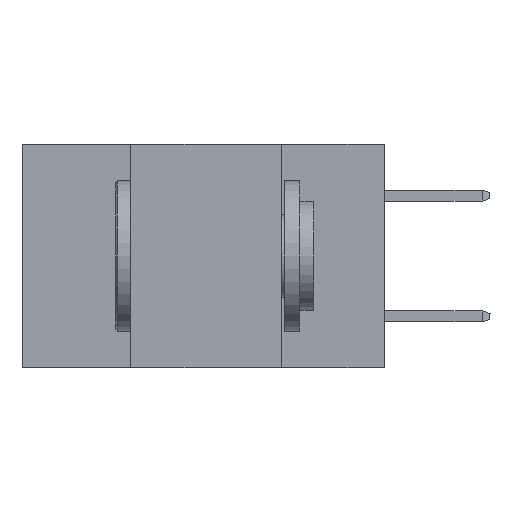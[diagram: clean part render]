
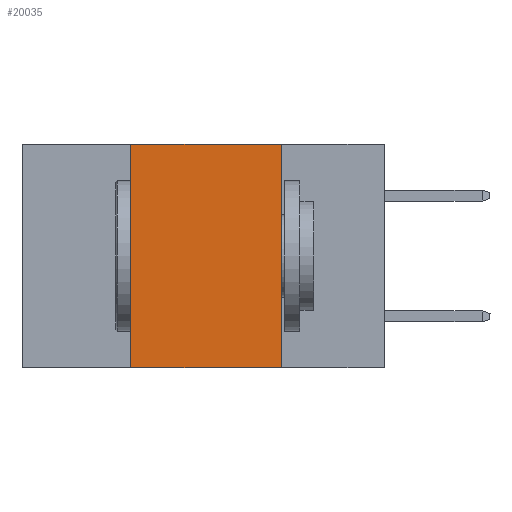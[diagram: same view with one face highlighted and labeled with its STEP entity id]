
A CAD part, left-side view. The second image highlights one B-rep face of the part: STEP entity #20035.
In plain terms, the highlighted planar face has unit normal (-1, 0, 0).
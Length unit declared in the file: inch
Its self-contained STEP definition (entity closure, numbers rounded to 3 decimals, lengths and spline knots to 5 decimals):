
#351 = VERTEX_POINT ( 'NONE', #7982 ) ;
#1203 = PLANE ( 'NONE',  #13184 ) ;
#2662 = DIRECTION ( 'NONE',  ( 0., 0., -1. ) ) ;
#3090 = CARTESIAN_POINT ( 'NONE',  ( 0., 0.6, 0. ) ) ;
#3167 = DIRECTION ( 'NONE',  ( 1., 0., 0. ) ) ;
#3627 = VERTEX_POINT ( 'NONE', #15160 ) ;
#3742 = CARTESIAN_POINT ( 'NONE',  ( 0., 0.6, 0. ) ) ;
#4454 = EDGE_CURVE ( 'NONE', #16259, #22683, #21124, .T. ) ;
#4916 = EDGE_LOOP ( 'NONE', ( #21546, #22739, #7546, #8337 ) ) ;
#5152 = CARTESIAN_POINT ( 'NONE',  ( 0., 0.42, 0. ) ) ;
#5723 = DIRECTION ( 'NONE',  ( 0., -1., 0. ) ) ;
#5740 = VECTOR ( 'NONE', #5723, 39.37008 ) ;
#6518 = CARTESIAN_POINT ( 'NONE',  ( 0., 0.17, 0. ) ) ;
#7094 = CARTESIAN_POINT ( 'NONE',  ( 0., 0.42, 0. ) ) ;
#7546 = ORIENTED_EDGE ( 'NONE', *, *, #14778, .F. ) ;
#7982 = CARTESIAN_POINT ( 'NONE',  ( 0., 0.42, -0.37 ) ) ;
#8337 = ORIENTED_EDGE ( 'NONE', *, *, #21241, .T. ) ;
#9645 = EDGE_CURVE ( 'NONE', #22683, #3627, #12155, .T. ) ;
#11070 = LINE ( 'NONE', #5152, #16207 ) ;
#12155 = LINE ( 'NONE', #16227, #12737 ) ;
#12737 = VECTOR ( 'NONE', #2662, 39.37008 ) ;
#13184 = AXIS2_PLACEMENT_3D ( 'NONE', #3090, #3167, #16722 ) ;
#14121 = CARTESIAN_POINT ( 'NONE',  ( 0., 0.6, -0.37 ) ) ;
#14778 = EDGE_CURVE ( 'NONE', #351, #16259, #11070, .T. ) ;
#15047 = LINE ( 'NONE', #14121, #20170 ) ;
#15160 = CARTESIAN_POINT ( 'NONE',  ( 0., 0.17, -0.37 ) ) ;
#16207 = VECTOR ( 'NONE', #18638, 39.37008 ) ;
#16227 = CARTESIAN_POINT ( 'NONE',  ( 0., 0.17, 0. ) ) ;
#16259 = VERTEX_POINT ( 'NONE', #7094 ) ;
#16722 = DIRECTION ( 'NONE',  ( 0., 0., -1. ) ) ;
#18173 = DIRECTION ( 'NONE',  ( 0., -1., 0. ) ) ;
#18638 = DIRECTION ( 'NONE',  ( 0., 0., 1. ) ) ;
#20035 = ADVANCED_FACE ( 'NONE', ( #22369 ), #1203, .F. ) ;
#20170 = VECTOR ( 'NONE', #18173, 39.37008 ) ;
#21124 = LINE ( 'NONE', #3742, #5740 ) ;
#21241 = EDGE_CURVE ( 'NONE', #351, #3627, #15047, .T. ) ;
#21546 = ORIENTED_EDGE ( 'NONE', *, *, #9645, .F. ) ;
#22369 = FACE_OUTER_BOUND ( 'NONE', #4916, .T. ) ;
#22683 = VERTEX_POINT ( 'NONE', #6518 ) ;
#22739 = ORIENTED_EDGE ( 'NONE', *, *, #4454, .F. ) ;
